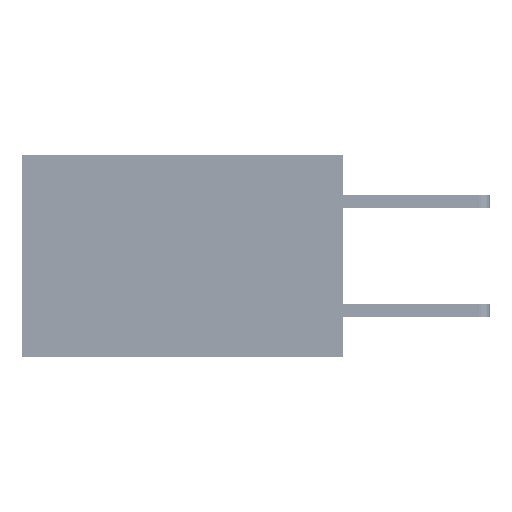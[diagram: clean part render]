
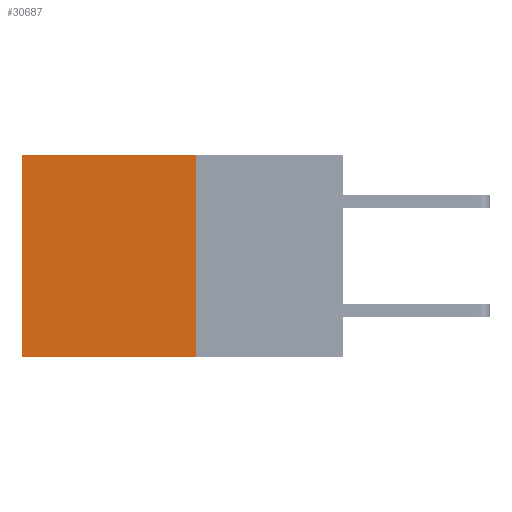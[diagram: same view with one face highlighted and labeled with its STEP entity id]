
A CAD part, left-side view. The second image highlights one B-rep face of the part: STEP entity #30687.
In plain terms, the highlighted planar face has unit normal (-1, 0, 0).
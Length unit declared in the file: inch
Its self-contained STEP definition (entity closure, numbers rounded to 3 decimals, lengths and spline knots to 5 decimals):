
#591 = VECTOR ( 'NONE', #33230, 39.37008 ) ;
#1156 = EDGE_LOOP ( 'NONE', ( #23308, #3768, #16047, #31588 ) ) ;
#1410 = LINE ( 'NONE', #30532, #591 ) ;
#2632 = CARTESIAN_POINT ( 'NONE',  ( 0.277, 0.59, 0. ) ) ;
#3010 = VECTOR ( 'NONE', #28664, 39.37008 ) ;
#3768 = ORIENTED_EDGE ( 'NONE', *, *, #27820, .F. ) ;
#6586 = DIRECTION ( 'NONE',  ( 0., 0., -1. ) ) ;
#6645 = CARTESIAN_POINT ( 'NONE',  ( 0.277, 0.59, -0.37 ) ) ;
#7297 = CARTESIAN_POINT ( 'NONE',  ( 0.277, 0.27, -0.37 ) ) ;
#8423 = EDGE_CURVE ( 'NONE', #21022, #10207, #19128, .T. ) ;
#8716 = CARTESIAN_POINT ( 'NONE',  ( 0.277, 0.27, 0. ) ) ;
#9070 = DIRECTION ( 'NONE',  ( 0., 0., -1. ) ) ;
#9086 = DIRECTION ( 'NONE',  ( 0., 0., -1. ) ) ;
#10151 = VERTEX_POINT ( 'NONE', #2632 ) ;
#10207 = VERTEX_POINT ( 'NONE', #21537 ) ;
#10448 = EDGE_CURVE ( 'NONE', #10151, #17539, #11428, .T. ) ;
#11428 = LINE ( 'NONE', #25068, #18565 ) ;
#13508 = AXIS2_PLACEMENT_3D ( 'NONE', #19975, #22649, #6586 ) ;
#16047 = ORIENTED_EDGE ( 'NONE', *, *, #8423, .F. ) ;
#16787 = EDGE_CURVE ( 'NONE', #21022, #10151, #1410, .T. ) ;
#17278 = PLANE ( 'NONE',  #13508 ) ;
#17539 = VERTEX_POINT ( 'NONE', #6645 ) ;
#18298 = VECTOR ( 'NONE', #9086, 39.37008 ) ;
#18565 = VECTOR ( 'NONE', #9070, 39.37008 ) ;
#19128 = LINE ( 'NONE', #19773, #18298 ) ;
#19773 = CARTESIAN_POINT ( 'NONE',  ( 0.277, 0.27, -0.37 ) ) ;
#19975 = CARTESIAN_POINT ( 'NONE',  ( 0.277, 0.27, -0.37 ) ) ;
#21022 = VERTEX_POINT ( 'NONE', #8716 ) ;
#21537 = CARTESIAN_POINT ( 'NONE',  ( 0.277, 0.27, -0.37 ) ) ;
#22649 = DIRECTION ( 'NONE',  ( 1., 0., 0. ) ) ;
#23308 = ORIENTED_EDGE ( 'NONE', *, *, #10448, .T. ) ;
#23562 = LINE ( 'NONE', #7297, #3010 ) ;
#25068 = CARTESIAN_POINT ( 'NONE',  ( 0.277, 0.59, -0.37 ) ) ;
#27531 = FACE_OUTER_BOUND ( 'NONE', #1156, .T. ) ;
#27820 = EDGE_CURVE ( 'NONE', #10207, #17539, #23562, .T. ) ;
#28664 = DIRECTION ( 'NONE',  ( 0., 1., 0. ) ) ;
#30532 = CARTESIAN_POINT ( 'NONE',  ( 0.277, 0.27, 0. ) ) ;
#30687 = ADVANCED_FACE ( 'NONE', ( #27531 ), #17278, .F. ) ;
#31588 = ORIENTED_EDGE ( 'NONE', *, *, #16787, .T. ) ;
#33230 = DIRECTION ( 'NONE',  ( 0., 1., 0. ) ) ;
